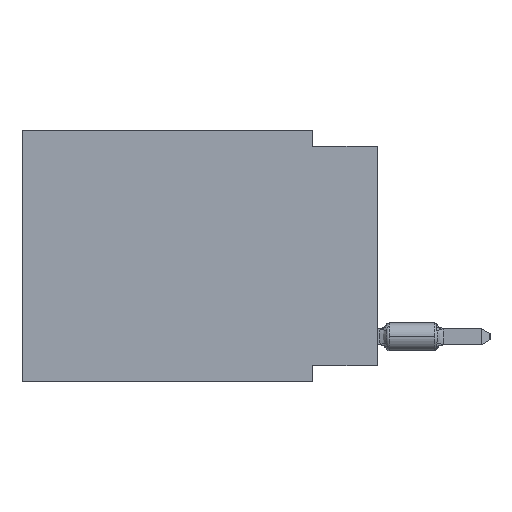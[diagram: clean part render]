
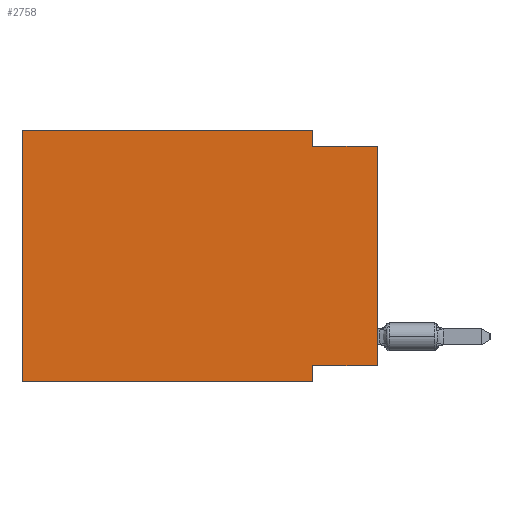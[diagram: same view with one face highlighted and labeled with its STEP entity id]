
A CAD part, left-side view. The second image highlights one B-rep face of the part: STEP entity #2758.
In plain terms, the highlighted planar face has unit normal (-1, 0, 0).
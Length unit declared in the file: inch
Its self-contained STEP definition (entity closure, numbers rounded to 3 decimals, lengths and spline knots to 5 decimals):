
#2758 = ADVANCED_FACE ( 'NONE', ( #12159 ), #36907, .F. ) ;
#2774 = CARTESIAN_POINT ( 'NONE',  ( 0., 0.1, -0.39 ) ) ;
#3170 = VECTOR ( 'NONE', #29675, 39.37008 ) ;
#3985 = CARTESIAN_POINT ( 'NONE',  ( 0., 0., -0.365 ) ) ;
#5231 = CARTESIAN_POINT ( 'NONE',  ( 0., 0.55, -0.39 ) ) ;
#7309 = VECTOR ( 'NONE', #59970, 39.37008 ) ;
#7636 = CARTESIAN_POINT ( 'NONE',  ( 0., 0.55, 0. ) ) ;
#8949 = CARTESIAN_POINT ( 'NONE',  ( 0., 0.1, -0.025 ) ) ;
#10935 = EDGE_CURVE ( 'NONE', #34919, #39330, #27345, .T. ) ;
#11795 = VECTOR ( 'NONE', #41872, 39.37008 ) ;
#12159 = FACE_OUTER_BOUND ( 'NONE', #34430, .T. ) ;
#12820 = ORIENTED_EDGE ( 'NONE', *, *, #46771, .F. ) ;
#13168 = DIRECTION ( 'NONE',  ( 0., 0., -1. ) ) ;
#14778 = LINE ( 'NONE', #61643, #11795 ) ;
#15104 = AXIS2_PLACEMENT_3D ( 'NONE', #22512, #21532, #27843 ) ;
#15305 = ORIENTED_EDGE ( 'NONE', *, *, #57632, .F. ) ;
#16451 = EDGE_CURVE ( 'NONE', #21072, #51516, #23695, .T. ) ;
#18005 = CARTESIAN_POINT ( 'NONE',  ( 0., 0., -0.025 ) ) ;
#18101 = CARTESIAN_POINT ( 'NONE',  ( 0., 0.1, 0. ) ) ;
#19679 = CARTESIAN_POINT ( 'NONE',  ( 0., 0., -0.365 ) ) ;
#21072 = VERTEX_POINT ( 'NONE', #8949 ) ;
#21532 = DIRECTION ( 'NONE',  ( 1., 0., 0. ) ) ;
#22512 = CARTESIAN_POINT ( 'NONE',  ( 0., 0.55, 0. ) ) ;
#22976 = DIRECTION ( 'NONE',  ( 0., -1., 0. ) ) ;
#23695 = LINE ( 'NONE', #18005, #44548 ) ;
#27345 = LINE ( 'NONE', #53156, #60613 ) ;
#27843 = DIRECTION ( 'NONE',  ( 0., 0., -1. ) ) ;
#28244 = CARTESIAN_POINT ( 'NONE',  ( 0., 0.1, -0.39 ) ) ;
#29023 = LINE ( 'NONE', #29354, #3170 ) ;
#29301 = ORIENTED_EDGE ( 'NONE', *, *, #33557, .F. ) ;
#29354 = CARTESIAN_POINT ( 'NONE',  ( 0., 0.55, 0. ) ) ;
#29471 = EDGE_CURVE ( 'NONE', #55007, #51516, #41205, .T. ) ;
#29675 = DIRECTION ( 'NONE',  ( 0., -1., 0. ) ) ;
#29868 = VERTEX_POINT ( 'NONE', #39473 ) ;
#30883 = ORIENTED_EDGE ( 'NONE', *, *, #46506, .F. ) ;
#30914 = CARTESIAN_POINT ( 'NONE',  ( 0., 0., -0.025 ) ) ;
#33102 = VECTOR ( 'NONE', #40066, 39.37008 ) ;
#33557 = EDGE_CURVE ( 'NONE', #34919, #55677, #14778, .T. ) ;
#33758 = ORIENTED_EDGE ( 'NONE', *, *, #16451, .F. ) ;
#34049 = DIRECTION ( 'NONE',  ( 0., -1., 0. ) ) ;
#34430 = EDGE_LOOP ( 'NONE', ( #49374, #33758, #12820, #15305, #29301, #63265, #30883, #46736 ) ) ;
#34919 = VERTEX_POINT ( 'NONE', #5231 ) ;
#36907 = PLANE ( 'NONE',  #15104 ) ;
#38937 = CARTESIAN_POINT ( 'NONE',  ( 0., 0.1, 0. ) ) ;
#39330 = VERTEX_POINT ( 'NONE', #28244 ) ;
#39473 = CARTESIAN_POINT ( 'NONE',  ( 0., 0.1, -0.365 ) ) ;
#40066 = DIRECTION ( 'NONE',  ( 0., 1., 0. ) ) ;
#41205 = LINE ( 'NONE', #61003, #44638 ) ;
#41872 = DIRECTION ( 'NONE',  ( 0., 0., 1. ) ) ;
#42019 = VERTEX_POINT ( 'NONE', #38937 ) ;
#44542 = LINE ( 'NONE', #18101, #7309 ) ;
#44548 = VECTOR ( 'NONE', #34049, 39.37008 ) ;
#44638 = VECTOR ( 'NONE', #61649, 39.37008 ) ;
#46506 = EDGE_CURVE ( 'NONE', #29868, #39330, #48664, .T. ) ;
#46736 = ORIENTED_EDGE ( 'NONE', *, *, #62981, .F. ) ;
#46771 = EDGE_CURVE ( 'NONE', #42019, #21072, #44542, .T. ) ;
#48664 = LINE ( 'NONE', #2774, #62859 ) ;
#49374 = ORIENTED_EDGE ( 'NONE', *, *, #29471, .T. ) ;
#51516 = VERTEX_POINT ( 'NONE', #30914 ) ;
#53156 = CARTESIAN_POINT ( 'NONE',  ( 0., 0.55, -0.39 ) ) ;
#55007 = VERTEX_POINT ( 'NONE', #3985 ) ;
#55677 = VERTEX_POINT ( 'NONE', #7636 ) ;
#57632 = EDGE_CURVE ( 'NONE', #55677, #42019, #29023, .T. ) ;
#59970 = DIRECTION ( 'NONE',  ( 0., 0., -1. ) ) ;
#60613 = VECTOR ( 'NONE', #22976, 39.37008 ) ;
#61003 = CARTESIAN_POINT ( 'NONE',  ( 0., 0., 0. ) ) ;
#61643 = CARTESIAN_POINT ( 'NONE',  ( 0., 0.55, 0. ) ) ;
#61649 = DIRECTION ( 'NONE',  ( 0., 0., 1. ) ) ;
#62859 = VECTOR ( 'NONE', #13168, 39.37008 ) ;
#62981 = EDGE_CURVE ( 'NONE', #55007, #29868, #66192, .T. ) ;
#63265 = ORIENTED_EDGE ( 'NONE', *, *, #10935, .T. ) ;
#66192 = LINE ( 'NONE', #19679, #33102 ) ;
